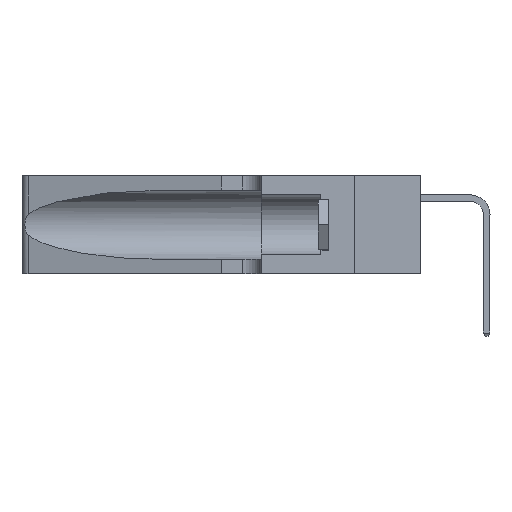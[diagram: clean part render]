
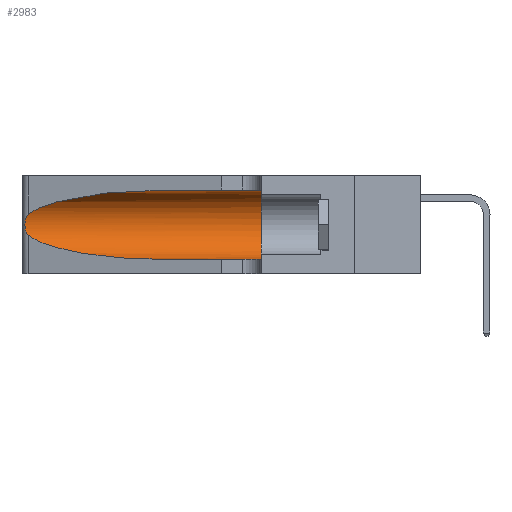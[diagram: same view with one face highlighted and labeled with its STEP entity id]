
A CAD part, left-side view. The second image highlights one B-rep face of the part: STEP entity #2983.
In plain terms, the highlighted cylindrical face has radius 3.308 mm (diameter 6.617 mm), a partial arc.
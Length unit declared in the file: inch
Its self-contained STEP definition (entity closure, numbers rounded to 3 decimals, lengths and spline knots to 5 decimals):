
#5 = CARTESIAN_POINT ( 'NONE',  ( 0.25789, 1.23486, 0.15765 ) ) ;
#1296 = CARTESIAN_POINT ( 'NONE',  ( 0.1305, 0.72297, 0.05475 ) ) ;
#2399 = CARTESIAN_POINT ( 'NONE',  ( 0.25487, 1.22718, 0.22369 ) ) ;
#2522 = CARTESIAN_POINT ( 'NONE',  ( 0.25555, 1.22993, 0.14849 ) ) ;
#2983 = ADVANCED_FACE ( 'NONE', ( #10334 ), #9542, .F. ) ;
#3012 = CARTESIAN_POINT ( 'NONE',  ( 0.1305, 0.35, 0.185 ) ) ;
#3720 = EDGE_CURVE ( 'NONE', #22797, #18680, #14248, .T. ) ;
#3838 = DIRECTION ( 'NONE',  ( 0., -1., 0. ) ) ;
#5538 = DIRECTION ( 'NONE',  ( 0., 0., 1. ) ) ;
#5809 = EDGE_CURVE ( 'NONE', #22764, #6542, #10830, .T. ) ;
#6542 = VERTEX_POINT ( 'NONE', #18595 ) ;
#7343 = CARTESIAN_POINT ( 'NONE',  ( 0.1305, 0.72297, 0.31525 ) ) ;
#7484 = CARTESIAN_POINT ( 'NONE',  ( 0.25787, 1.23484, 0.2124 ) ) ;
#8205 = CARTESIAN_POINT ( 'NONE',  ( 0.18966, 0.96281, 0.31525 ) ) ;
#8888 = ORIENTED_EDGE ( 'NONE', *, *, #5809, .T. ) ;
#9542 = CYLINDRICAL_SURFACE ( 'NONE', #29505, 0.13025 ) ;
#9618 = ORIENTED_EDGE ( 'NONE', *, *, #3720, .T. ) ;
#9639 = EDGE_LOOP ( 'NONE', ( #8888, #11807, #9618, #13397, #27793, #12922 ) ) ;
#10065 = CARTESIAN_POINT ( 'NONE',  ( 0.26018, 1.23835, 0.19895 ) ) ;
#10334 = FACE_OUTER_BOUND ( 'NONE', #9639, .T. ) ;
#10524 = DIRECTION ( 'NONE',  ( 0., -1., 0. ) ) ;
#10830 =( BOUNDED_CURVE ( )  B_SPLINE_CURVE ( 3, ( #13307, #8205, #23354, #30888 ),
 .UNSPECIFIED., .F., .T. ) 
 B_SPLINE_CURVE_WITH_KNOTS ( ( 4, 4 ),
 ( 1.5708, 2.84003 ),
 .UNSPECIFIED. ) 
 CURVE ( )  GEOMETRIC_REPRESENTATION_ITEM ( )  RATIONAL_B_SPLINE_CURVE ( ( 1., 0.87, 0.87, 1. ) ) 
 REPRESENTATION_ITEM ( '' )  );
#11086 = CARTESIAN_POINT ( 'NONE',  ( 0.1305, 0.35, 0.31525 ) ) ;
#11484 = CARTESIAN_POINT ( 'NONE',  ( 0.1305, 1.61858, 0.31525 ) ) ;
#11510 = DIRECTION ( 'NONE',  ( 0., 0., -1. ) ) ;
#11807 = ORIENTED_EDGE ( 'NONE', *, *, #27156, .T. ) ;
#12326 = CARTESIAN_POINT ( 'NONE',  ( 0.1305, 0.72297, 0.05475 ) ) ;
#12592 = CARTESIAN_POINT ( 'NONE',  ( 0.26075, 1.23896, 0.178 ) ) ;
#12922 = ORIENTED_EDGE ( 'NONE', *, *, #25653, .F. ) ;
#13070 = EDGE_CURVE ( 'NONE', #20554, #28907, #16641, .T. ) ;
#13307 = CARTESIAN_POINT ( 'NONE',  ( 0.1305, 0.72297, 0.31525 ) ) ;
#13314 = VECTOR ( 'NONE', #16455, 39.37008 ) ;
#13397 = ORIENTED_EDGE ( 'NONE', *, *, #26735, .T. ) ;
#14248 =( BOUNDED_CURVE ( )  B_SPLINE_CURVE ( 3, ( #27450, #19861, #22399, #12326 ),
 .UNSPECIFIED., .F., .F. ) 
 B_SPLINE_CURVE_WITH_KNOTS ( ( 4, 4 ),
 ( 3.44316, 4.71239 ),
 .UNSPECIFIED. ) 
 CURVE ( )  GEOMETRIC_REPRESENTATION_ITEM ( )  RATIONAL_B_SPLINE_CURVE ( ( 1., 0.87, 0.87, 1. ) ) 
 REPRESENTATION_ITEM ( '' )  );
#14727 = CARTESIAN_POINT ( 'NONE',  ( 0.1305, 0.35, 0.05475 ) ) ;
#15152 = CARTESIAN_POINT ( 'NONE',  ( 0.25856, 1.23593, 0.16098 ) ) ;
#15590 = B_SPLINE_CURVE_WITH_KNOTS ( 'NONE', 3,
 ( #2399, #20135, #22643, #7484, #25195, #10065, #27713, #12592, #30198, #15152, #5, #17707, #2522, #20242 ),
 .UNSPECIFIED., .F., .F.,
 ( 4, 2, 2, 2, 2, 2, 4 ),
 ( 0., 0.00027, 0.00053, 0.00107, 0.0016, 0.00187, 0.00214 ),
 .UNSPECIFIED. ) ;
#16455 = DIRECTION ( 'NONE',  ( 0., -1., 0. ) ) ;
#16581 = CARTESIAN_POINT ( 'NONE',  ( 0.1305, 1.61858, 0.185 ) ) ;
#16641 = CIRCLE ( 'NONE', #29086, 0.13025 ) ;
#17707 = CARTESIAN_POINT ( 'NONE',  ( 0.25639, 1.23186, 0.15144 ) ) ;
#18595 = CARTESIAN_POINT ( 'NONE',  ( 0.25487, 1.22718, 0.22369 ) ) ;
#18680 = VERTEX_POINT ( 'NONE', #1296 ) ;
#19861 = CARTESIAN_POINT ( 'NONE',  ( 0.2373, 1.15595, 0.08982 ) ) ;
#20135 = CARTESIAN_POINT ( 'NONE',  ( 0.25555, 1.22994, 0.2215 ) ) ;
#20205 = CARTESIAN_POINT ( 'NONE',  ( 0.25487, 1.22718, 0.14631 ) ) ;
#20242 = CARTESIAN_POINT ( 'NONE',  ( 0.25487, 1.22718, 0.14631 ) ) ;
#20554 = VERTEX_POINT ( 'NONE', #11086 ) ;
#20753 = DIRECTION ( 'NONE',  ( 0., 1., 0. ) ) ;
#20857 = LINE ( 'NONE', #11484, #13314 ) ;
#21169 = VECTOR ( 'NONE', #10524, 39.37008 ) ;
#22399 = CARTESIAN_POINT ( 'NONE',  ( 0.18966, 0.96281, 0.05475 ) ) ;
#22643 = CARTESIAN_POINT ( 'NONE',  ( 0.25639, 1.23184, 0.21858 ) ) ;
#22764 = VERTEX_POINT ( 'NONE', #7343 ) ;
#22797 = VERTEX_POINT ( 'NONE', #20205 ) ;
#23113 = CARTESIAN_POINT ( 'NONE',  ( 0.1305, 1.61858, 0.05475 ) ) ;
#23354 = CARTESIAN_POINT ( 'NONE',  ( 0.2373, 1.15595, 0.28018 ) ) ;
#25195 = CARTESIAN_POINT ( 'NONE',  ( 0.25854, 1.2359, 0.20912 ) ) ;
#25653 = EDGE_CURVE ( 'NONE', #22764, #20554, #20857, .T. ) ;
#26735 = EDGE_CURVE ( 'NONE', #18680, #28907, #27844, .T. ) ;
#27156 = EDGE_CURVE ( 'NONE', #6542, #22797, #15590, .T. ) ;
#27450 = CARTESIAN_POINT ( 'NONE',  ( 0.25487, 1.22718, 0.14631 ) ) ;
#27713 = CARTESIAN_POINT ( 'NONE',  ( 0.26075, 1.23896, 0.19203 ) ) ;
#27793 = ORIENTED_EDGE ( 'NONE', *, *, #13070, .F. ) ;
#27844 = LINE ( 'NONE', #23113, #21169 ) ;
#28907 = VERTEX_POINT ( 'NONE', #14727 ) ;
#29086 = AXIS2_PLACEMENT_3D ( 'NONE', #3012, #20753, #5538 ) ;
#29505 = AXIS2_PLACEMENT_3D ( 'NONE', #16581, #3838, #11510 ) ;
#30198 = CARTESIAN_POINT ( 'NONE',  ( 0.26017, 1.23833, 0.17102 ) ) ;
#30888 = CARTESIAN_POINT ( 'NONE',  ( 0.25487, 1.22718, 0.22369 ) ) ;
